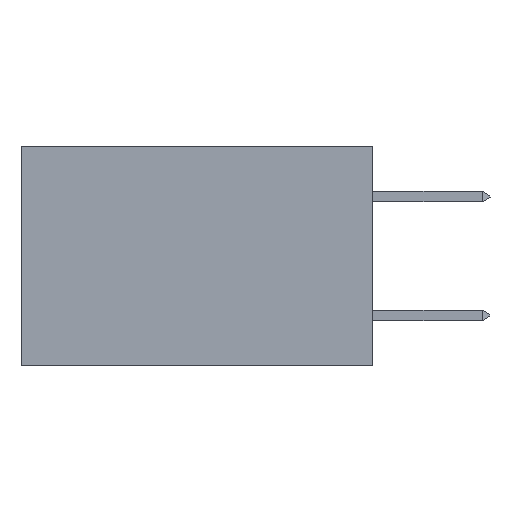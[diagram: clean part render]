
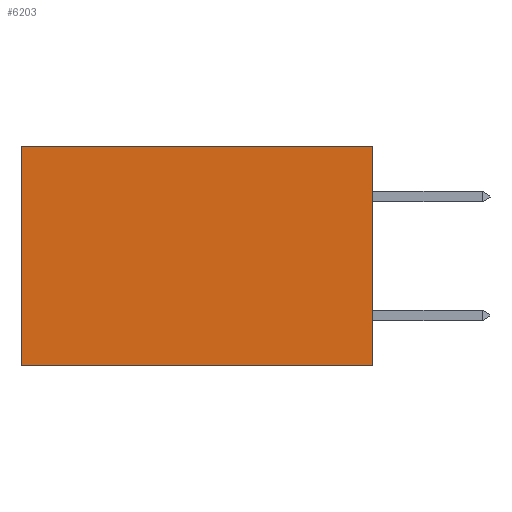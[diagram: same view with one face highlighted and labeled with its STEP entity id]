
A CAD part, left-side view. The second image highlights one B-rep face of the part: STEP entity #6203.
In plain terms, the highlighted planar face has unit normal (-1, 0, 0).
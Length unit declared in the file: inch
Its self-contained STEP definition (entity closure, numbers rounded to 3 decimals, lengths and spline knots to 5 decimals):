
#65 = EDGE_CURVE ( 'NONE', #6277, #7246, #11593, .T. ) ;
#219 = DIRECTION ( 'NONE',  ( 0., 1., 0. ) ) ;
#310 = CARTESIAN_POINT ( 'NONE',  ( 0.277, 0., -0.37 ) ) ;
#663 = DIRECTION ( 'NONE',  ( 0., 0., -1. ) ) ;
#794 = DIRECTION ( 'NONE',  ( 1., 0., 0. ) ) ;
#807 = CARTESIAN_POINT ( 'NONE',  ( 0.277, 0., -0.37 ) ) ;
#921 = PLANE ( 'NONE',  #3015 ) ;
#1692 = CARTESIAN_POINT ( 'NONE',  ( 0.277, 0., -0.37 ) ) ;
#2163 = ORIENTED_EDGE ( 'NONE', *, *, #5390, .F. ) ;
#2635 = LINE ( 'NONE', #310, #5288 ) ;
#2786 = VERTEX_POINT ( 'NONE', #1692 ) ;
#2788 = ORIENTED_EDGE ( 'NONE', *, *, #5254, .F. ) ;
#2897 = CARTESIAN_POINT ( 'NONE',  ( 0.277, 0.59, -0.37 ) ) ;
#3015 = AXIS2_PLACEMENT_3D ( 'NONE', #807, #794, #663 ) ;
#3301 = VERTEX_POINT ( 'NONE', #9147 ) ;
#3413 = VECTOR ( 'NONE', #7968, 39.37008 ) ;
#4523 = ORIENTED_EDGE ( 'NONE', *, *, #12607, .T. ) ;
#5254 = EDGE_CURVE ( 'NONE', #6277, #2786, #2635, .T. ) ;
#5288 = VECTOR ( 'NONE', #12837, 39.37008 ) ;
#5390 = EDGE_CURVE ( 'NONE', #2786, #3301, #11558, .T. ) ;
#5434 = ORIENTED_EDGE ( 'NONE', *, *, #65, .T. ) ;
#5953 = VECTOR ( 'NONE', #219, 39.37008 ) ;
#6203 = ADVANCED_FACE ( 'NONE', ( #6848 ), #921, .F. ) ;
#6277 = VERTEX_POINT ( 'NONE', #11890 ) ;
#6848 = FACE_OUTER_BOUND ( 'NONE', #9081, .T. ) ;
#7000 = VECTOR ( 'NONE', #10948, 39.37008 ) ;
#7246 = VERTEX_POINT ( 'NONE', #8014 ) ;
#7968 = DIRECTION ( 'NONE',  ( 0., 0., -1. ) ) ;
#8014 = CARTESIAN_POINT ( 'NONE',  ( 0.277, 0.59, 0. ) ) ;
#9081 = EDGE_LOOP ( 'NONE', ( #4523, #2163, #2788, #5434 ) ) ;
#9147 = CARTESIAN_POINT ( 'NONE',  ( 0.277, 0.59, -0.37 ) ) ;
#10948 = DIRECTION ( 'NONE',  ( 0., 1., 0. ) ) ;
#10949 = CARTESIAN_POINT ( 'NONE',  ( 0.277, 0., -0.37 ) ) ;
#11352 = LINE ( 'NONE', #2897, #3413 ) ;
#11558 = LINE ( 'NONE', #10949, #7000 ) ;
#11593 = LINE ( 'NONE', #11897, #5953 ) ;
#11890 = CARTESIAN_POINT ( 'NONE',  ( 0.277, 0., 0. ) ) ;
#11897 = CARTESIAN_POINT ( 'NONE',  ( 0.277, 0., 0. ) ) ;
#12607 = EDGE_CURVE ( 'NONE', #7246, #3301, #11352, .T. ) ;
#12837 = DIRECTION ( 'NONE',  ( 0., 0., -1. ) ) ;
